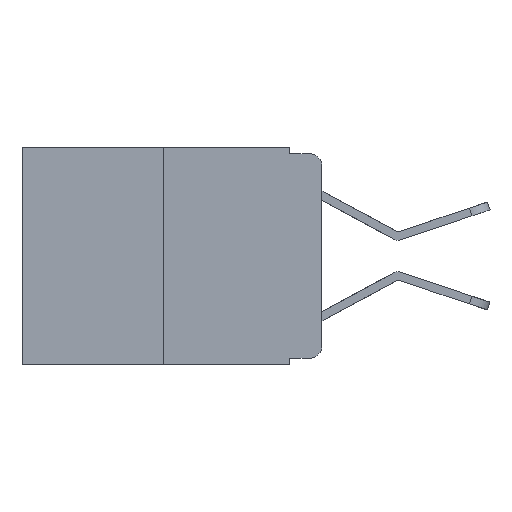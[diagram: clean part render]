
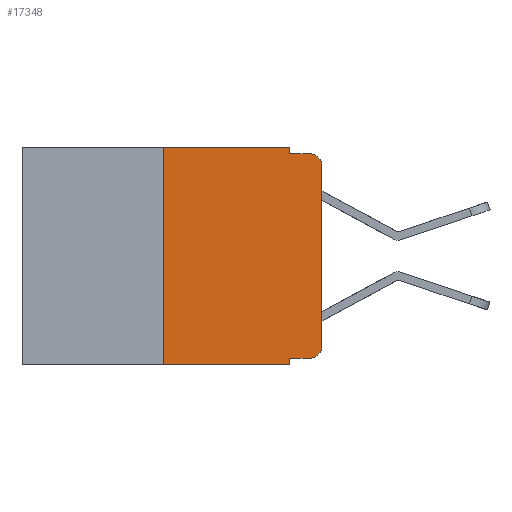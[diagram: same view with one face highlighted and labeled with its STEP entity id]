
A CAD part, left-side view. The second image highlights one B-rep face of the part: STEP entity #17348.
In plain terms, the highlighted planar face has unit normal (-1, 0, 0).
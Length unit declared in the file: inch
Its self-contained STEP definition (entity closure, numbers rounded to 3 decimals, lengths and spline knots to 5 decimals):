
#167 = EDGE_CURVE ( 'NONE', #1155, #18629, #7960, .T. ) ;
#331 = VECTOR ( 'NONE', #7998, 39.37008 ) ;
#450 = LINE ( 'NONE', #11370, #6056 ) ;
#546 = DIRECTION ( 'NONE',  ( 0., 0., 1. ) ) ;
#762 = ORIENTED_EDGE ( 'NONE', *, *, #6007, .F. ) ;
#918 = EDGE_CURVE ( 'NONE', #18629, #2865, #8958, .T. ) ;
#1120 = VERTEX_POINT ( 'NONE', #14269 ) ;
#1155 = VERTEX_POINT ( 'NONE', #14661 ) ;
#1343 = VECTOR ( 'NONE', #17476, 39.37008 ) ;
#1434 = CARTESIAN_POINT ( 'NONE',  ( 0., 0.051, -0.333 ) ) ;
#1762 = LINE ( 'NONE', #11156, #12635 ) ;
#1860 = DIRECTION ( 'NONE',  ( 0., 0., -1. ) ) ;
#1978 = VERTEX_POINT ( 'NONE', #17383 ) ;
#2266 = DIRECTION ( 'NONE',  ( 0., -1., 0. ) ) ;
#2364 = LINE ( 'NONE', #12869, #8677 ) ;
#2772 = DIRECTION ( 'NONE',  ( -1., 0., 0. ) ) ;
#2865 = VERTEX_POINT ( 'NONE', #17726 ) ;
#3074 = DIRECTION ( 'NONE',  ( 0., 0., -1. ) ) ;
#3460 = AXIS2_PLACEMENT_3D ( 'NONE', #10748, #2772, #3074 ) ;
#3589 = ORIENTED_EDGE ( 'NONE', *, *, #11146, .T. ) ;
#3639 = DIRECTION ( 'NONE',  ( 0., 0., -1. ) ) ;
#3724 = ORIENTED_EDGE ( 'NONE', *, *, #17708, .T. ) ;
#4052 = VERTEX_POINT ( 'NONE', #15334 ) ;
#5118 = DIRECTION ( 'NONE',  ( 0., 0., 1. ) ) ;
#5209 = CARTESIAN_POINT ( 'NONE',  ( 0., 0., -0.03 ) ) ;
#5216 = CIRCLE ( 'NONE', #10384, 0.02 ) ;
#5713 = EDGE_LOOP ( 'NONE', ( #10070, #19356, #762, #14933, #19044, #10413, #8669, #17207, #3589, #3724 ) ) ;
#5783 = DIRECTION ( 'NONE',  ( 0., 0., -1. ) ) ;
#5892 = DIRECTION ( 'NONE',  ( 1., 0., 0. ) ) ;
#5978 = CARTESIAN_POINT ( 'NONE',  ( 0., 0.051, 0. ) ) ;
#6007 = EDGE_CURVE ( 'NONE', #16932, #2865, #450, .T. ) ;
#6056 = VECTOR ( 'NONE', #2266, 39.37008 ) ;
#6377 = LINE ( 'NONE', #11138, #331 ) ;
#6883 = DIRECTION ( 'NONE',  ( -1., 0., 0. ) ) ;
#7198 = DIRECTION ( 'NONE',  ( 0., -1., 0. ) ) ;
#7708 = DIRECTION ( 'NONE',  ( 0., 0., -1. ) ) ;
#7960 = LINE ( 'NONE', #17309, #12095 ) ;
#7998 = DIRECTION ( 'NONE',  ( 0., -1., 0. ) ) ;
#8669 = ORIENTED_EDGE ( 'NONE', *, *, #16359, .T. ) ;
#8672 = VERTEX_POINT ( 'NONE', #18249 ) ;
#8677 = VECTOR ( 'NONE', #546, 39.37008 ) ;
#8916 = FACE_OUTER_BOUND ( 'NONE', #5713, .T. ) ;
#8958 = CIRCLE ( 'NONE', #3460, 0.02 ) ;
#9890 = EDGE_CURVE ( 'NONE', #11204, #16932, #10214, .T. ) ;
#10070 = ORIENTED_EDGE ( 'NONE', *, *, #167, .T. ) ;
#10214 = LINE ( 'NONE', #5978, #16022 ) ;
#10331 = PLANE ( 'NONE',  #15525 ) ;
#10384 = AXIS2_PLACEMENT_3D ( 'NONE', #17855, #6883, #3639 ) ;
#10413 = ORIENTED_EDGE ( 'NONE', *, *, #13017, .F. ) ;
#10748 = CARTESIAN_POINT ( 'NONE',  ( 0., 0.02, -0.03 ) ) ;
#11138 = CARTESIAN_POINT ( 'NONE',  ( 0., 0.473, -0.343 ) ) ;
#11146 = EDGE_CURVE ( 'NONE', #1120, #8672, #18282, .T. ) ;
#11156 = CARTESIAN_POINT ( 'NONE',  ( 0., 0.051, 0. ) ) ;
#11204 = VERTEX_POINT ( 'NONE', #15064 ) ;
#11370 = CARTESIAN_POINT ( 'NONE',  ( 0., 0.051, -0.01 ) ) ;
#11452 = VERTEX_POINT ( 'NONE', #13793 ) ;
#11859 = VECTOR ( 'NONE', #7198, 39.37008 ) ;
#12095 = VECTOR ( 'NONE', #5118, 39.37008 ) ;
#12172 = CARTESIAN_POINT ( 'NONE',  ( 0., 0.051, -0.01 ) ) ;
#12635 = VECTOR ( 'NONE', #1860, 39.37008 ) ;
#12661 = LINE ( 'NONE', #14283, #1343 ) ;
#12869 = CARTESIAN_POINT ( 'NONE',  ( 0., 0.25, 0. ) ) ;
#13017 = EDGE_CURVE ( 'NONE', #4052, #11452, #2364, .T. ) ;
#13793 = CARTESIAN_POINT ( 'NONE',  ( 0., 0.25, 0. ) ) ;
#14269 = CARTESIAN_POINT ( 'NONE',  ( 0., 0.051, -0.333 ) ) ;
#14283 = CARTESIAN_POINT ( 'NONE',  ( 0., 0.473, 0. ) ) ;
#14661 = CARTESIAN_POINT ( 'NONE',  ( 0., 0., -0.313 ) ) ;
#14933 = ORIENTED_EDGE ( 'NONE', *, *, #9890, .F. ) ;
#15064 = CARTESIAN_POINT ( 'NONE',  ( 0., 0.051, 0. ) ) ;
#15334 = CARTESIAN_POINT ( 'NONE',  ( 0., 0.25, -0.343 ) ) ;
#15525 = AXIS2_PLACEMENT_3D ( 'NONE', #18387, #5892, #7708 ) ;
#15855 = EDGE_CURVE ( 'NONE', #1120, #1978, #1762, .T. ) ;
#16022 = VECTOR ( 'NONE', #5783, 39.37008 ) ;
#16359 = EDGE_CURVE ( 'NONE', #4052, #1978, #6377, .T. ) ;
#16932 = VERTEX_POINT ( 'NONE', #12172 ) ;
#17142 = EDGE_CURVE ( 'NONE', #11452, #11204, #12661, .T. ) ;
#17207 = ORIENTED_EDGE ( 'NONE', *, *, #15855, .F. ) ;
#17309 = CARTESIAN_POINT ( 'NONE',  ( 0., 0., 0. ) ) ;
#17348 = ADVANCED_FACE ( 'NONE', ( #8916 ), #10331, .F. ) ;
#17383 = CARTESIAN_POINT ( 'NONE',  ( 0., 0.051, -0.343 ) ) ;
#17476 = DIRECTION ( 'NONE',  ( 0., -1., 0. ) ) ;
#17708 = EDGE_CURVE ( 'NONE', #8672, #1155, #5216, .T. ) ;
#17726 = CARTESIAN_POINT ( 'NONE',  ( 0., 0.02, -0.01 ) ) ;
#17855 = CARTESIAN_POINT ( 'NONE',  ( 0., 0.02, -0.313 ) ) ;
#18249 = CARTESIAN_POINT ( 'NONE',  ( 0., 0.02, -0.333 ) ) ;
#18282 = LINE ( 'NONE', #1434, #11859 ) ;
#18387 = CARTESIAN_POINT ( 'NONE',  ( 0., 0.473, 0. ) ) ;
#18629 = VERTEX_POINT ( 'NONE', #5209 ) ;
#19044 = ORIENTED_EDGE ( 'NONE', *, *, #17142, .F. ) ;
#19356 = ORIENTED_EDGE ( 'NONE', *, *, #918, .T. ) ;
